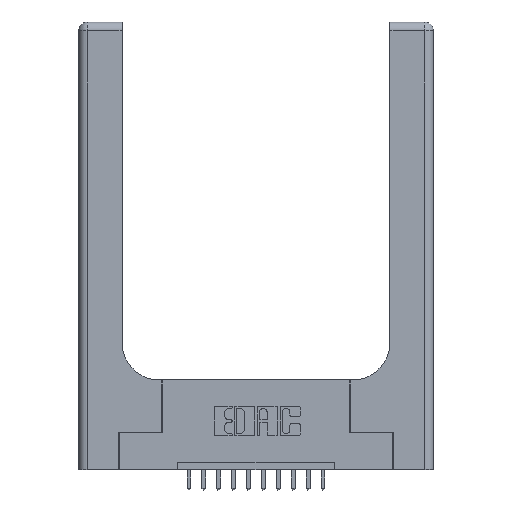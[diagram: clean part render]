
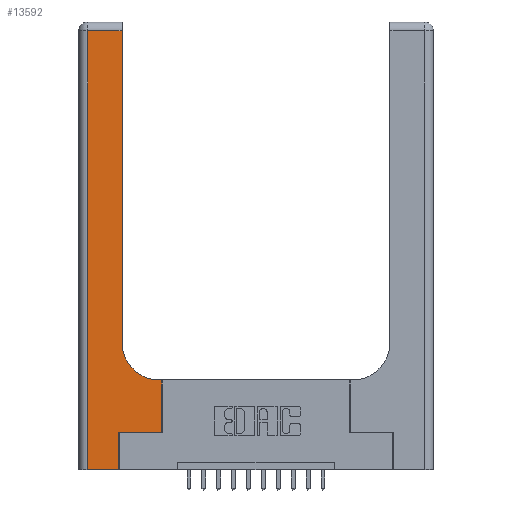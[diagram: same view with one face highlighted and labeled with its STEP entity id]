
A CAD part, top view. The second image highlights one B-rep face of the part: STEP entity #13592.
In plain terms, the highlighted planar face has unit normal (0, 0, 1).
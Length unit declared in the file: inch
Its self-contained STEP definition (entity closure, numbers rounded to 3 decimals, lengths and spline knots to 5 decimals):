
#213 = DIRECTION ( 'NONE',  ( 0., 0., -1. ) ) ;
#992 = DIRECTION ( 'NONE',  ( 1., 0., 0. ) ) ;
#1533 = ORIENTED_EDGE ( 'NONE', *, *, #8339, .T. ) ;
#1950 = AXIS2_PLACEMENT_3D ( 'NONE', #16445, #6005, #11337 ) ;
#2185 = EDGE_CURVE ( 'NONE', #14849, #9115, #10881, .T. ) ;
#2653 = DIRECTION ( 'NONE',  ( 0., 1., 0. ) ) ;
#2771 = ORIENTED_EDGE ( 'NONE', *, *, #10927, .T. ) ;
#2837 = DIRECTION ( 'NONE',  ( 0., -1., 0. ) ) ;
#3057 = CARTESIAN_POINT ( 'NONE',  ( 0.06, 3., 0.37 ) ) ;
#3599 = LINE ( 'NONE', #9161, #15525 ) ;
#3607 = DIRECTION ( 'NONE',  ( 1., 0., 0. ) ) ;
#3635 = CARTESIAN_POINT ( 'NONE',  ( 0.5585, 0.25, 0.37 ) ) ;
#3661 = LINE ( 'NONE', #8857, #6115 ) ;
#3983 = DIRECTION ( 'NONE',  ( -1., 0., 0. ) ) ;
#4226 = VECTOR ( 'NONE', #3983, 39.37008 ) ;
#4538 = EDGE_CURVE ( 'NONE', #6656, #7735, #9145, .T. ) ;
#4575 = EDGE_CURVE ( 'NONE', #12643, #17013, #5671, .T. ) ;
#4615 = ORIENTED_EDGE ( 'NONE', *, *, #2185, .T. ) ;
#4909 = CIRCLE ( 'NONE', #1950, 0.25 ) ;
#5100 = CARTESIAN_POINT ( 'NONE',  ( 0.5585, 0.6, 0.37 ) ) ;
#5324 = EDGE_CURVE ( 'NONE', #7735, #7270, #3599, .T. ) ;
#5625 = CARTESIAN_POINT ( 'NONE',  ( 0.269, 0., 0.37 ) ) ;
#5671 = LINE ( 'NONE', #13000, #4226 ) ;
#6005 = DIRECTION ( 'NONE',  ( 0., 0., -1. ) ) ;
#6087 = ORIENTED_EDGE ( 'NONE', *, *, #9580, .T. ) ;
#6102 = VERTEX_POINT ( 'NONE', #15956 ) ;
#6115 = VECTOR ( 'NONE', #992, 39.37008 ) ;
#6252 = VECTOR ( 'NONE', #15386, 39.37008 ) ;
#6633 = AXIS2_PLACEMENT_3D ( 'NONE', #12105, #213, #14897 ) ;
#6656 = VERTEX_POINT ( 'NONE', #12933 ) ;
#7201 = LINE ( 'NONE', #7311, #11699 ) ;
#7270 = VERTEX_POINT ( 'NONE', #10551 ) ;
#7311 = CARTESIAN_POINT ( 'NONE',  ( 0.2915, 0.6, 0.37 ) ) ;
#7505 = CARTESIAN_POINT ( 'NONE',  ( 0., 0., 0.37 ) ) ;
#7552 = CARTESIAN_POINT ( 'NONE',  ( 0.2915, 3., 0.37 ) ) ;
#7735 = VERTEX_POINT ( 'NONE', #5625 ) ;
#8339 = EDGE_CURVE ( 'NONE', #9115, #12481, #7201, .T. ) ;
#8486 = CARTESIAN_POINT ( 'NONE',  ( 0.2915, 2.94, 0.37 ) ) ;
#8738 = VECTOR ( 'NONE', #2837, 39.37008 ) ;
#8857 = CARTESIAN_POINT ( 'NONE',  ( 0.269, 0.25, 0.37 ) ) ;
#8878 = FACE_OUTER_BOUND ( 'NONE', #11352, .T. ) ;
#8924 = ORIENTED_EDGE ( 'NONE', *, *, #5324, .T. ) ;
#9115 = VERTEX_POINT ( 'NONE', #5100 ) ;
#9145 = LINE ( 'NONE', #7505, #14521 ) ;
#9161 = CARTESIAN_POINT ( 'NONE',  ( 0.269, 0., 0.37 ) ) ;
#9205 = ORIENTED_EDGE ( 'NONE', *, *, #16785, .T. ) ;
#9338 = LINE ( 'NONE', #3057, #8738 ) ;
#9580 = EDGE_CURVE ( 'NONE', #7270, #14849, #3661, .T. ) ;
#9631 = DIRECTION ( 'NONE',  ( -1., 0., 0. ) ) ;
#9754 = CARTESIAN_POINT ( 'NONE',  ( 0.06, 2.94, 0.37 ) ) ;
#10551 = CARTESIAN_POINT ( 'NONE',  ( 0.269, 0.25, 0.37 ) ) ;
#10674 = DIRECTION ( 'NONE',  ( 0., 1., 0. ) ) ;
#10881 = LINE ( 'NONE', #16020, #14611 ) ;
#10927 = EDGE_CURVE ( 'NONE', #17013, #6656, #9338, .T. ) ;
#11337 = DIRECTION ( 'NONE',  ( 1., 0., 0. ) ) ;
#11352 = EDGE_LOOP ( 'NONE', ( #12323, #12714, #2771, #16924, #8924, #6087, #4615, #1533, #9205 ) ) ;
#11570 = EDGE_CURVE ( 'NONE', #6102, #12643, #14129, .T. ) ;
#11699 = VECTOR ( 'NONE', #9631, 39.37008 ) ;
#12105 = CARTESIAN_POINT ( 'NONE',  ( 0., 3., 0.37 ) ) ;
#12221 = PLANE ( 'NONE',  #6633 ) ;
#12323 = ORIENTED_EDGE ( 'NONE', *, *, #11570, .T. ) ;
#12481 = VERTEX_POINT ( 'NONE', #16767 ) ;
#12643 = VERTEX_POINT ( 'NONE', #8486 ) ;
#12714 = ORIENTED_EDGE ( 'NONE', *, *, #4575, .T. ) ;
#12933 = CARTESIAN_POINT ( 'NONE',  ( 0.06, 0., 0.37 ) ) ;
#13000 = CARTESIAN_POINT ( 'NONE',  ( 0., 2.94, 0.37 ) ) ;
#13592 = ADVANCED_FACE ( 'NONE', ( #8878 ), #12221, .F. ) ;
#14129 = LINE ( 'NONE', #7552, #6252 ) ;
#14521 = VECTOR ( 'NONE', #3607, 39.37008 ) ;
#14611 = VECTOR ( 'NONE', #10674, 39.37008 ) ;
#14849 = VERTEX_POINT ( 'NONE', #3635 ) ;
#14897 = DIRECTION ( 'NONE',  ( -1., 0., 0. ) ) ;
#15386 = DIRECTION ( 'NONE',  ( 0., 1., 0. ) ) ;
#15525 = VECTOR ( 'NONE', #2653, 39.37008 ) ;
#15956 = CARTESIAN_POINT ( 'NONE',  ( 0.2915, 0.85, 0.37 ) ) ;
#16020 = CARTESIAN_POINT ( 'NONE',  ( 0.5585, 0.25, 0.37 ) ) ;
#16445 = CARTESIAN_POINT ( 'NONE',  ( 0.5415, 0.85, 0.37 ) ) ;
#16767 = CARTESIAN_POINT ( 'NONE',  ( 0.5415, 0.6, 0.37 ) ) ;
#16785 = EDGE_CURVE ( 'NONE', #12481, #6102, #4909, .T. ) ;
#16924 = ORIENTED_EDGE ( 'NONE', *, *, #4538, .T. ) ;
#17013 = VERTEX_POINT ( 'NONE', #9754 ) ;
